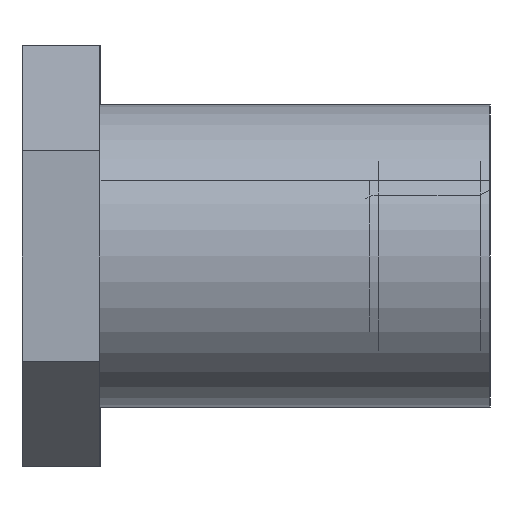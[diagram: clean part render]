
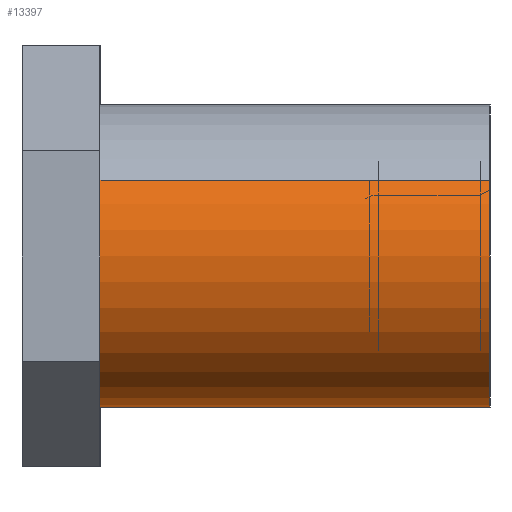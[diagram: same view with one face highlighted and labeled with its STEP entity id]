
A CAD part, left-side view. The second image highlights one B-rep face of the part: STEP entity #13397.
In plain terms, the highlighted cylindrical face has radius 1.968 mm (diameter 3.937 mm), a partial arc.
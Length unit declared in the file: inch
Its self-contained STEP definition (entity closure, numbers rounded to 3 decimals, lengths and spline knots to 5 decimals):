
#45 = AXIS2_PLACEMENT_3D ( 'NONE', #23028, #22528, #10896 ) ;
#115 = LINE ( 'NONE', #13767, #3910 ) ;
#1081 = CARTESIAN_POINT ( 'NONE',  ( 0., 0.24, -0.0775 ) ) ;
#1553 = CARTESIAN_POINT ( 'NONE',  ( 0., 0.24, 0.0775 ) ) ;
#1629 = CARTESIAN_POINT ( 'NONE',  ( 0., 0.04, -0.0775 ) ) ;
#2136 = CIRCLE ( 'NONE', #45, 0.0775 ) ;
#3283 = CIRCLE ( 'NONE', #4102, 0.0775 ) ;
#3910 = VECTOR ( 'NONE', #12063, 39.37008 ) ;
#4102 = AXIS2_PLACEMENT_3D ( 'NONE', #21424, #17288, #23764 ) ;
#4562 = ORIENTED_EDGE ( 'NONE', *, *, #6893, .T. ) ;
#4759 = ORIENTED_EDGE ( 'NONE', *, *, #13639, .F. ) ;
#4949 = CARTESIAN_POINT ( 'NONE',  ( 0., 0.04, 0.0775 ) ) ;
#5337 = LINE ( 'NONE', #15094, #17377 ) ;
#6180 = EDGE_LOOP ( 'NONE', ( #6195, #4759, #23578, #4562 ) ) ;
#6195 = ORIENTED_EDGE ( 'NONE', *, *, #20917, .F. ) ;
#6893 = EDGE_CURVE ( 'NONE', #9805, #7276, #3283, .T. ) ;
#7276 = VERTEX_POINT ( 'NONE', #4949 ) ;
#9805 = VERTEX_POINT ( 'NONE', #1629 ) ;
#10896 = DIRECTION ( 'NONE',  ( 0., 0., 1. ) ) ;
#11802 = DIRECTION ( 'NONE',  ( 0., -1., 0. ) ) ;
#12063 = DIRECTION ( 'NONE',  ( 0., -1., 0. ) ) ;
#13397 = ADVANCED_FACE ( 'NONE', ( #19701 ), #19575, .T. ) ;
#13639 = EDGE_CURVE ( 'NONE', #17650, #25592, #2136, .T. ) ;
#13767 = CARTESIAN_POINT ( 'NONE',  ( 0., 0.24, -0.0775 ) ) ;
#15050 = AXIS2_PLACEMENT_3D ( 'NONE', #25266, #11802, #17624 ) ;
#15094 = CARTESIAN_POINT ( 'NONE',  ( 0., 0.24, 0.0775 ) ) ;
#17063 = EDGE_CURVE ( 'NONE', #17650, #9805, #115, .T. ) ;
#17288 = DIRECTION ( 'NONE',  ( 0., 1., 0. ) ) ;
#17377 = VECTOR ( 'NONE', #22962, 39.37008 ) ;
#17624 = DIRECTION ( 'NONE',  ( 0., 0., -1. ) ) ;
#17650 = VERTEX_POINT ( 'NONE', #1081 ) ;
#19575 = CYLINDRICAL_SURFACE ( 'NONE', #15050, 0.0775 ) ;
#19701 = FACE_OUTER_BOUND ( 'NONE', #6180, .T. ) ;
#20917 = EDGE_CURVE ( 'NONE', #25592, #7276, #5337, .T. ) ;
#21424 = CARTESIAN_POINT ( 'NONE',  ( 0., 0.04, 0. ) ) ;
#22528 = DIRECTION ( 'NONE',  ( 0., 1., 0. ) ) ;
#22962 = DIRECTION ( 'NONE',  ( 0., -1., 0. ) ) ;
#23028 = CARTESIAN_POINT ( 'NONE',  ( 0., 0.24, 0. ) ) ;
#23578 = ORIENTED_EDGE ( 'NONE', *, *, #17063, .T. ) ;
#23764 = DIRECTION ( 'NONE',  ( 0., 0., 1. ) ) ;
#25266 = CARTESIAN_POINT ( 'NONE',  ( 0., 0.24, 0. ) ) ;
#25592 = VERTEX_POINT ( 'NONE', #1553 ) ;
